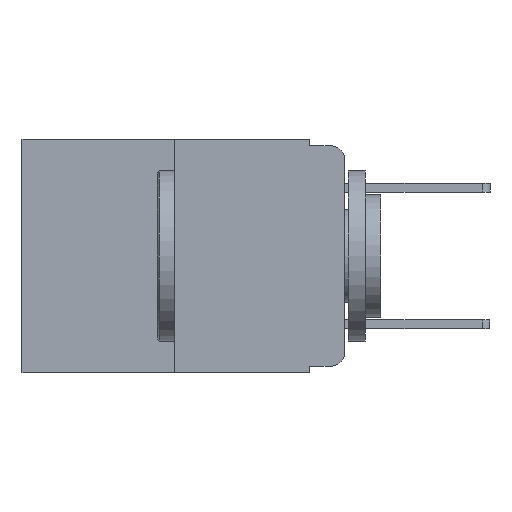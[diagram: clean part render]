
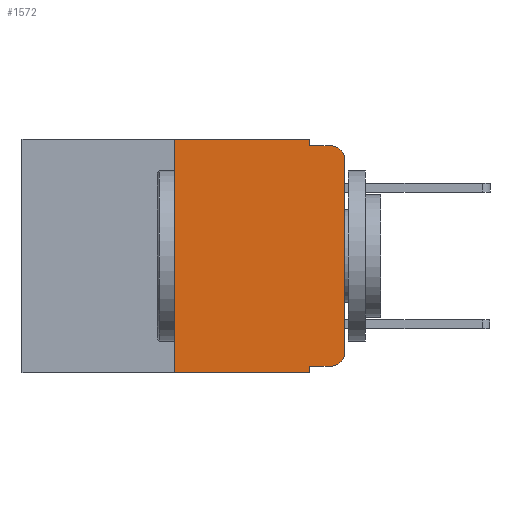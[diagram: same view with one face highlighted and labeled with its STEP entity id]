
A CAD part, left-side view. The second image highlights one B-rep face of the part: STEP entity #1572.
In plain terms, the highlighted planar face has unit normal (-1, 0, 0).
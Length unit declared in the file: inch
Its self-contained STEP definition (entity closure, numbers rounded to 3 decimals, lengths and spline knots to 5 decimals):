
#49 = CARTESIAN_POINT ( 'NONE',  ( 0., 0.051, 0. ) ) ;
#194 = EDGE_LOOP ( 'NONE', ( #4877, #5245, #1696, #7922, #7535, #7074, #8836, #8400, #7500, #5261 ) ) ;
#256 = CARTESIAN_POINT ( 'NONE',  ( 0., 0.051, 0. ) ) ;
#414 = AXIS2_PLACEMENT_3D ( 'NONE', #8608, #8889, #5137 ) ;
#581 = LINE ( 'NONE', #3310, #2677 ) ;
#599 = CARTESIAN_POINT ( 'NONE',  ( 0., 0., 0. ) ) ;
#650 = PLANE ( 'NONE',  #414 ) ;
#854 = VERTEX_POINT ( 'NONE', #4786 ) ;
#861 = EDGE_CURVE ( 'NONE', #854, #3119, #2929, .T. ) ;
#977 = VERTEX_POINT ( 'NONE', #4950 ) ;
#990 = FACE_OUTER_BOUND ( 'NONE', #194, .T. ) ;
#1156 = CARTESIAN_POINT ( 'NONE',  ( 0., 0.02, -0.313 ) ) ;
#1208 = EDGE_CURVE ( 'NONE', #977, #5025, #1712, .T. ) ;
#1348 = AXIS2_PLACEMENT_3D ( 'NONE', #4755, #2017, #5477 ) ;
#1572 = ADVANCED_FACE ( 'NONE', ( #990 ), #650, .F. ) ;
#1696 = ORIENTED_EDGE ( 'NONE', *, *, #8842, .F. ) ;
#1712 = LINE ( 'NONE', #10465, #9918 ) ;
#1880 = LINE ( 'NONE', #2757, #4104 ) ;
#1944 = EDGE_CURVE ( 'NONE', #9923, #977, #5435, .T. ) ;
#2017 = DIRECTION ( 'NONE',  ( -1., 0., 0. ) ) ;
#2178 = DIRECTION ( 'NONE',  ( 0., -1., 0. ) ) ;
#2242 = DIRECTION ( 'NONE',  ( 0., 0., 1. ) ) ;
#2456 = VECTOR ( 'NONE', #2178, 39.37008 ) ;
#2659 = LINE ( 'NONE', #49, #8979 ) ;
#2677 = VECTOR ( 'NONE', #3921, 39.37008 ) ;
#2715 = CARTESIAN_POINT ( 'NONE',  ( 0., 0.25, 0. ) ) ;
#2757 = CARTESIAN_POINT ( 'NONE',  ( 0., 0.051, -0.01 ) ) ;
#2868 = EDGE_CURVE ( 'NONE', #3119, #10338, #7530, .T. ) ;
#2929 = LINE ( 'NONE', #3723, #8754 ) ;
#3119 = VERTEX_POINT ( 'NONE', #10276 ) ;
#3310 = CARTESIAN_POINT ( 'NONE',  ( 0., 0.051, 0. ) ) ;
#3322 = VECTOR ( 'NONE', #9820, 39.37008 ) ;
#3361 = CARTESIAN_POINT ( 'NONE',  ( 0., 0., -0.313 ) ) ;
#3403 = EDGE_CURVE ( 'NONE', #9923, #10298, #4621, .T. ) ;
#3419 = CARTESIAN_POINT ( 'NONE',  ( 0., 0., -0.03 ) ) ;
#3523 = CARTESIAN_POINT ( 'NONE',  ( 0., 0.02, -0.01 ) ) ;
#3723 = CARTESIAN_POINT ( 'NONE',  ( 0., 0.051, -0.333 ) ) ;
#3894 = EDGE_CURVE ( 'NONE', #4620, #6841, #4130, .T. ) ;
#3921 = DIRECTION ( 'NONE',  ( 0., 0., -1. ) ) ;
#4104 = VECTOR ( 'NONE', #8344, 39.37008 ) ;
#4130 = CIRCLE ( 'NONE', #1348, 0.02 ) ;
#4620 = VERTEX_POINT ( 'NONE', #3419 ) ;
#4621 = LINE ( 'NONE', #6359, #2456 ) ;
#4755 = CARTESIAN_POINT ( 'NONE',  ( 0., 0.02, -0.03 ) ) ;
#4786 = CARTESIAN_POINT ( 'NONE',  ( 0., 0.051, -0.333 ) ) ;
#4815 = DIRECTION ( 'NONE',  ( 0., -1., 0. ) ) ;
#4877 = ORIENTED_EDGE ( 'NONE', *, *, #7119, .T. ) ;
#4950 = CARTESIAN_POINT ( 'NONE',  ( 0., 0.25, 0. ) ) ;
#5025 = VERTEX_POINT ( 'NONE', #256 ) ;
#5137 = DIRECTION ( 'NONE',  ( 0., 0., -1. ) ) ;
#5174 = DIRECTION ( 'NONE',  ( 0., 0., -1. ) ) ;
#5226 = DIRECTION ( 'NONE',  ( 0., 0., -1. ) ) ;
#5245 = ORIENTED_EDGE ( 'NONE', *, *, #3894, .T. ) ;
#5261 = ORIENTED_EDGE ( 'NONE', *, *, #2868, .T. ) ;
#5435 = LINE ( 'NONE', #2715, #3322 ) ;
#5477 = DIRECTION ( 'NONE',  ( 0., 0., -1. ) ) ;
#6267 = EDGE_CURVE ( 'NONE', #5025, #7670, #581, .T. ) ;
#6359 = CARTESIAN_POINT ( 'NONE',  ( 0., 0.473, -0.343 ) ) ;
#6516 = DIRECTION ( 'NONE',  ( 0., -1., 0. ) ) ;
#6793 = LINE ( 'NONE', #599, #9047 ) ;
#6841 = VERTEX_POINT ( 'NONE', #3523 ) ;
#6852 = CARTESIAN_POINT ( 'NONE',  ( 0., 0.051, -0.01 ) ) ;
#7074 = ORIENTED_EDGE ( 'NONE', *, *, #1944, .F. ) ;
#7119 = EDGE_CURVE ( 'NONE', #10338, #4620, #6793, .T. ) ;
#7500 = ORIENTED_EDGE ( 'NONE', *, *, #861, .T. ) ;
#7530 = CIRCLE ( 'NONE', #8749, 0.02 ) ;
#7535 = ORIENTED_EDGE ( 'NONE', *, *, #1208, .F. ) ;
#7670 = VERTEX_POINT ( 'NONE', #6852 ) ;
#7922 = ORIENTED_EDGE ( 'NONE', *, *, #6267, .F. ) ;
#8200 = CARTESIAN_POINT ( 'NONE',  ( 0., 0.25, -0.343 ) ) ;
#8344 = DIRECTION ( 'NONE',  ( 0., -1., 0. ) ) ;
#8400 = ORIENTED_EDGE ( 'NONE', *, *, #10021, .F. ) ;
#8608 = CARTESIAN_POINT ( 'NONE',  ( 0., 0.473, 0. ) ) ;
#8749 = AXIS2_PLACEMENT_3D ( 'NONE', #1156, #10020, #5226 ) ;
#8754 = VECTOR ( 'NONE', #6516, 39.37008 ) ;
#8836 = ORIENTED_EDGE ( 'NONE', *, *, #3403, .T. ) ;
#8842 = EDGE_CURVE ( 'NONE', #7670, #6841, #1880, .T. ) ;
#8889 = DIRECTION ( 'NONE',  ( 1., 0., 0. ) ) ;
#8979 = VECTOR ( 'NONE', #5174, 39.37008 ) ;
#9047 = VECTOR ( 'NONE', #2242, 39.37008 ) ;
#9554 = CARTESIAN_POINT ( 'NONE',  ( 0., 0.051, -0.343 ) ) ;
#9820 = DIRECTION ( 'NONE',  ( 0., 0., 1. ) ) ;
#9918 = VECTOR ( 'NONE', #4815, 39.37008 ) ;
#9923 = VERTEX_POINT ( 'NONE', #8200 ) ;
#10020 = DIRECTION ( 'NONE',  ( -1., 0., 0. ) ) ;
#10021 = EDGE_CURVE ( 'NONE', #854, #10298, #2659, .T. ) ;
#10276 = CARTESIAN_POINT ( 'NONE',  ( 0., 0.02, -0.333 ) ) ;
#10298 = VERTEX_POINT ( 'NONE', #9554 ) ;
#10338 = VERTEX_POINT ( 'NONE', #3361 ) ;
#10465 = CARTESIAN_POINT ( 'NONE',  ( 0., 0.473, 0. ) ) ;
